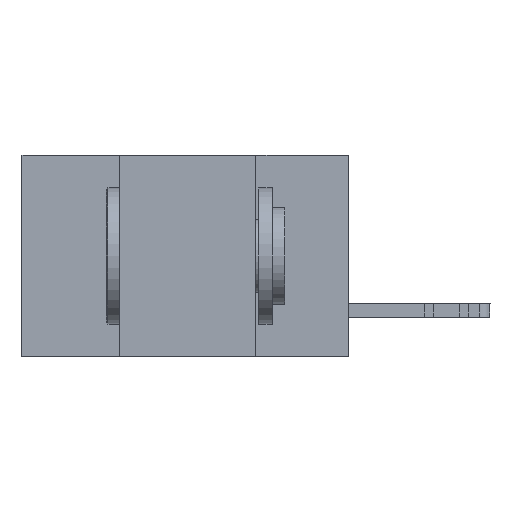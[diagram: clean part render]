
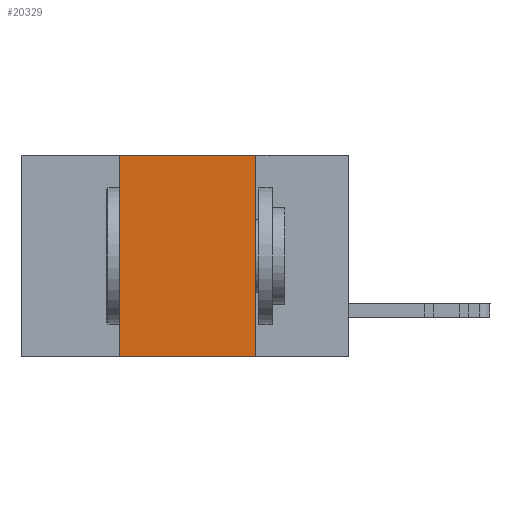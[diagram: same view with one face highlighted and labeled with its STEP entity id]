
A CAD part, left-side view. The second image highlights one B-rep face of the part: STEP entity #20329.
In plain terms, the highlighted planar face has unit normal (-1, 0, 0).
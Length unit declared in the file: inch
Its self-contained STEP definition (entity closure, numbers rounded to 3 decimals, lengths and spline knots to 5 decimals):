
#907 = CARTESIAN_POINT ( 'NONE',  ( 0., 0.17, 0. ) ) ;
#994 = CARTESIAN_POINT ( 'NONE',  ( 0., 0.6, 0. ) ) ;
#2105 = VERTEX_POINT ( 'NONE', #15787 ) ;
#2294 = VECTOR ( 'NONE', #25750, 39.37008 ) ;
#3103 = EDGE_CURVE ( 'NONE', #19159, #12808, #27555, .T. ) ;
#3110 = LINE ( 'NONE', #3486, #18417 ) ;
#3486 = CARTESIAN_POINT ( 'NONE',  ( 0., 0.17, 0. ) ) ;
#5550 = LINE ( 'NONE', #10149, #29936 ) ;
#5562 = CARTESIAN_POINT ( 'NONE',  ( 0., 0.42, 0. ) ) ;
#5802 = DIRECTION ( 'NONE',  ( 0., 0., -1. ) ) ;
#6065 = FACE_OUTER_BOUND ( 'NONE', #28844, .T. ) ;
#7174 = EDGE_CURVE ( 'NONE', #2105, #19159, #31367, .T. ) ;
#7507 = CARTESIAN_POINT ( 'NONE',  ( 0., 0.6, 0. ) ) ;
#9817 = CARTESIAN_POINT ( 'NONE',  ( 0., 0.17, -0.37 ) ) ;
#10149 = CARTESIAN_POINT ( 'NONE',  ( 0., 0.6, -0.37 ) ) ;
#11172 = PLANE ( 'NONE',  #11869 ) ;
#11869 = AXIS2_PLACEMENT_3D ( 'NONE', #994, #20857, #5802 ) ;
#12808 = VERTEX_POINT ( 'NONE', #907 ) ;
#13227 = ORIENTED_EDGE ( 'NONE', *, *, #29805, .T. ) ;
#13413 = ORIENTED_EDGE ( 'NONE', *, *, #3103, .F. ) ;
#15165 = DIRECTION ( 'NONE',  ( 0., -1., 0. ) ) ;
#15754 = VECTOR ( 'NONE', #22655, 39.37008 ) ;
#15787 = CARTESIAN_POINT ( 'NONE',  ( 0., 0.42, -0.37 ) ) ;
#16735 = EDGE_CURVE ( 'NONE', #12808, #19009, #3110, .T. ) ;
#18417 = VECTOR ( 'NONE', #23565, 39.37008 ) ;
#19009 = VERTEX_POINT ( 'NONE', #9817 ) ;
#19159 = VERTEX_POINT ( 'NONE', #25958 ) ;
#19654 = ORIENTED_EDGE ( 'NONE', *, *, #7174, .F. ) ;
#20329 = ADVANCED_FACE ( 'NONE', ( #6065 ), #11172, .F. ) ;
#20857 = DIRECTION ( 'NONE',  ( 1., 0., 0. ) ) ;
#21874 = ORIENTED_EDGE ( 'NONE', *, *, #16735, .F. ) ;
#22655 = DIRECTION ( 'NONE',  ( 0., -1., 0. ) ) ;
#23565 = DIRECTION ( 'NONE',  ( 0., 0., -1. ) ) ;
#25750 = DIRECTION ( 'NONE',  ( 0., 0., 1. ) ) ;
#25958 = CARTESIAN_POINT ( 'NONE',  ( 0., 0.42, 0. ) ) ;
#27555 = LINE ( 'NONE', #7507, #15754 ) ;
#28844 = EDGE_LOOP ( 'NONE', ( #21874, #13413, #19654, #13227 ) ) ;
#29805 = EDGE_CURVE ( 'NONE', #2105, #19009, #5550, .T. ) ;
#29936 = VECTOR ( 'NONE', #15165, 39.37008 ) ;
#31367 = LINE ( 'NONE', #5562, #2294 ) ;
